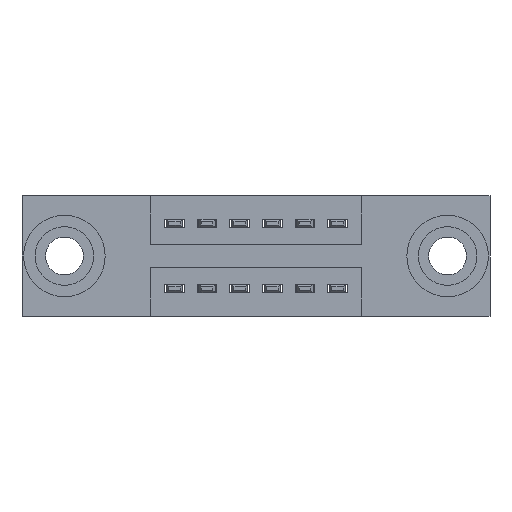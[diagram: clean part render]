
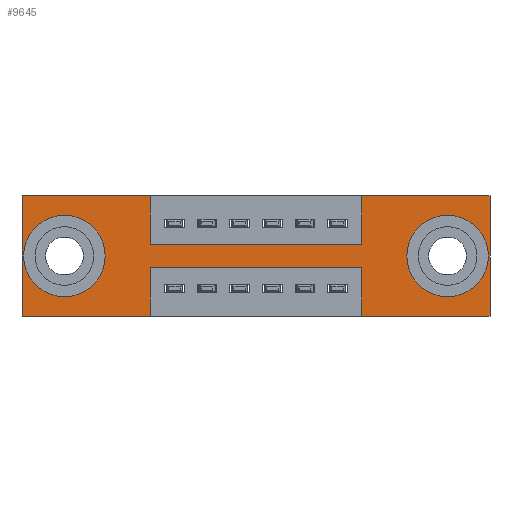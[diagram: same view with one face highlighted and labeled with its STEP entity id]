
A CAD part, front view. The second image highlights one B-rep face of the part: STEP entity #9645.
In plain terms, the highlighted planar face has unit normal (0, -1, 0).
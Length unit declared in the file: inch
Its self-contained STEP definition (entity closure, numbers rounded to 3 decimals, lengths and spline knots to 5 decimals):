
#14 = VERTEX_POINT ( 'NONE', #7489 ) ;
#21 = VECTOR ( 'NONE', #7703, 39.37008 ) ;
#127 = VERTEX_POINT ( 'NONE', #4537 ) ;
#397 = LINE ( 'NONE', #4495, #6055 ) ;
#702 = CARTESIAN_POINT ( 'NONE',  ( 0., 0., -0.37 ) ) ;
#749 = VECTOR ( 'NONE', #4626, 39.37008 ) ;
#845 = DIRECTION ( 'NONE',  ( 0., 0., 1. ) ) ;
#919 = DIRECTION ( 'NONE',  ( 0., 1., 0. ) ) ;
#989 = VERTEX_POINT ( 'NONE', #2778 ) ;
#1026 = LINE ( 'NONE', #3140, #4791 ) ;
#1046 = DIRECTION ( 'NONE',  ( 0., 0., -1. ) ) ;
#1113 = LINE ( 'NONE', #6927, #8847 ) ;
#1201 = DIRECTION ( 'NONE',  ( 0., 0., -1. ) ) ;
#1492 = ORIENTED_EDGE ( 'NONE', *, *, #8970, .F. ) ;
#1616 = VECTOR ( 'NONE', #5543, 39.37008 ) ;
#1700 = FACE_BOUND ( 'NONE', #3421, .T. ) ;
#1702 = ORIENTED_EDGE ( 'NONE', *, *, #8540, .T. ) ;
#1722 = CIRCLE ( 'NONE', #2268, 0.078 ) ;
#1865 = AXIS2_PLACEMENT_3D ( 'NONE', #5554, #919, #6311 ) ;
#1942 = PLANE ( 'NONE',  #3237 ) ;
#2005 = VERTEX_POINT ( 'NONE', #9450 ) ;
#2013 = AXIS2_PLACEMENT_3D ( 'NONE', #4120, #4902, #1046 ) ;
#2085 = CARTESIAN_POINT ( 'NONE',  ( 0., 0., 0. ) ) ;
#2108 = LINE ( 'NONE', #3737, #1616 ) ;
#2268 = AXIS2_PLACEMENT_3D ( 'NONE', #8088, #8887, #4190 ) ;
#2319 = DIRECTION ( 'NONE',  ( 0., 0., -1. ) ) ;
#2701 = VECTOR ( 'NONE', #6085, 39.37008 ) ;
#2749 = DIRECTION ( 'NONE',  ( 0., -1., 0. ) ) ;
#2778 = CARTESIAN_POINT ( 'NONE',  ( 1.435, 0., -0.37 ) ) ;
#2894 = ORIENTED_EDGE ( 'NONE', *, *, #7302, .F. ) ;
#3048 = EDGE_CURVE ( 'NONE', #7345, #127, #9031, .T. ) ;
#3110 = CARTESIAN_POINT ( 'NONE',  ( 0.13, 0., -0.263 ) ) ;
#3140 = CARTESIAN_POINT ( 'NONE',  ( 1.0425, 0., 0. ) ) ;
#3148 = FACE_BOUND ( 'NONE', #8759, .T. ) ;
#3237 = AXIS2_PLACEMENT_3D ( 'NONE', #5823, #2749, #1201 ) ;
#3384 = LINE ( 'NONE', #7835, #21 ) ;
#3421 = EDGE_LOOP ( 'NONE', ( #7200, #1702 ) ) ;
#3453 = CARTESIAN_POINT ( 'NONE',  ( 1.0425, 0., -0.22 ) ) ;
#3467 = CARTESIAN_POINT ( 'NONE',  ( 0., 0., 0. ) ) ;
#3473 = EDGE_CURVE ( 'NONE', #2005, #4674, #1026, .T. ) ;
#3604 = EDGE_CURVE ( 'NONE', #127, #7345, #7560, .T. ) ;
#3635 = CARTESIAN_POINT ( 'NONE',  ( 1.0425, 0., 0. ) ) ;
#3707 = CARTESIAN_POINT ( 'NONE',  ( 1.305, 0., -0.185 ) ) ;
#3736 = CARTESIAN_POINT ( 'NONE',  ( 0.3925, 0., -0.15 ) ) ;
#3737 = CARTESIAN_POINT ( 'NONE',  ( 0., 0., 0. ) ) ;
#3738 = DIRECTION ( 'NONE',  ( 0., 0., -1. ) ) ;
#3801 = VERTEX_POINT ( 'NONE', #10041 ) ;
#3845 = CARTESIAN_POINT ( 'NONE',  ( 0.3925, 0., 0. ) ) ;
#3860 = VERTEX_POINT ( 'NONE', #5006 ) ;
#3964 = ORIENTED_EDGE ( 'NONE', *, *, #8935, .F. ) ;
#4093 = ORIENTED_EDGE ( 'NONE', *, *, #7135, .F. ) ;
#4120 = CARTESIAN_POINT ( 'NONE',  ( 1.305, 0., -0.185 ) ) ;
#4127 = CARTESIAN_POINT ( 'NONE',  ( 1.435, 0., 0. ) ) ;
#4190 = DIRECTION ( 'NONE',  ( 0., 0., 1. ) ) ;
#4197 = CARTESIAN_POINT ( 'NONE',  ( 0.3925, 0., 0. ) ) ;
#4222 = ORIENTED_EDGE ( 'NONE', *, *, #7178, .F. ) ;
#4417 = VECTOR ( 'NONE', #6828, 39.37008 ) ;
#4495 = CARTESIAN_POINT ( 'NONE',  ( 1.435, 0., 0. ) ) ;
#4537 = CARTESIAN_POINT ( 'NONE',  ( 1.305, 0., -0.263 ) ) ;
#4626 = DIRECTION ( 'NONE',  ( 0., 0., -1. ) ) ;
#4647 = EDGE_CURVE ( 'NONE', #3801, #2005, #6429, .T. ) ;
#4674 = VERTEX_POINT ( 'NONE', #3635 ) ;
#4726 = ORIENTED_EDGE ( 'NONE', *, *, #3048, .T. ) ;
#4761 = LINE ( 'NONE', #10022, #2701 ) ;
#4791 = VECTOR ( 'NONE', #845, 39.37008 ) ;
#4902 = DIRECTION ( 'NONE',  ( 0., 1., 0. ) ) ;
#5006 = CARTESIAN_POINT ( 'NONE',  ( 0.3925, 0., -0.22 ) ) ;
#5101 = EDGE_CURVE ( 'NONE', #6743, #7125, #5962, .T. ) ;
#5230 = VERTEX_POINT ( 'NONE', #3110 ) ;
#5314 = EDGE_CURVE ( 'NONE', #989, #9769, #9468, .T. ) ;
#5410 = ORIENTED_EDGE ( 'NONE', *, *, #9427, .F. ) ;
#5413 = EDGE_CURVE ( 'NONE', #3860, #6776, #1113, .T. ) ;
#5426 = ORIENTED_EDGE ( 'NONE', *, *, #5413, .F. ) ;
#5447 = FACE_OUTER_BOUND ( 'NONE', #8054, .T. ) ;
#5543 = DIRECTION ( 'NONE',  ( 0., 0., 1. ) ) ;
#5551 = ORIENTED_EDGE ( 'NONE', *, *, #3604, .T. ) ;
#5554 = CARTESIAN_POINT ( 'NONE',  ( 0.13, 0., -0.185 ) ) ;
#5560 = CARTESIAN_POINT ( 'NONE',  ( 1.305, 0., -0.107 ) ) ;
#5597 = VECTOR ( 'NONE', #7647, 39.37008 ) ;
#5735 = CIRCLE ( 'NONE', #1865, 0.078 ) ;
#5823 = CARTESIAN_POINT ( 'NONE',  ( 0., 0., -0.37 ) ) ;
#5962 = LINE ( 'NONE', #3467, #9977 ) ;
#6055 = VECTOR ( 'NONE', #9184, 39.37008 ) ;
#6085 = DIRECTION ( 'NONE',  ( 0., 0., 1. ) ) ;
#6293 = VECTOR ( 'NONE', #7999, 39.37008 ) ;
#6311 = DIRECTION ( 'NONE',  ( 0., 0., 1. ) ) ;
#6429 = LINE ( 'NONE', #3736, #4417 ) ;
#6546 = CARTESIAN_POINT ( 'NONE',  ( 0.13, 0., -0.107 ) ) ;
#6661 = LINE ( 'NONE', #3845, #749 ) ;
#6692 = LINE ( 'NONE', #9579, #7045 ) ;
#6732 = CARTESIAN_POINT ( 'NONE',  ( 0., 0., 0. ) ) ;
#6743 = VERTEX_POINT ( 'NONE', #2085 ) ;
#6776 = VERTEX_POINT ( 'NONE', #9772 ) ;
#6828 = DIRECTION ( 'NONE',  ( 1., 0., 0. ) ) ;
#6927 = CARTESIAN_POINT ( 'NONE',  ( 0.3925, 0., -0.37 ) ) ;
#6940 = ORIENTED_EDGE ( 'NONE', *, *, #3473, .F. ) ;
#7045 = VECTOR ( 'NONE', #7358, 39.37008 ) ;
#7106 = EDGE_CURVE ( 'NONE', #9655, #5230, #5735, .T. ) ;
#7125 = VERTEX_POINT ( 'NONE', #4197 ) ;
#7135 = EDGE_CURVE ( 'NONE', #6776, #14, #6692, .T. ) ;
#7178 = EDGE_CURVE ( 'NONE', #14, #6743, #2108, .T. ) ;
#7200 = ORIENTED_EDGE ( 'NONE', *, *, #7106, .T. ) ;
#7265 = DIRECTION ( 'NONE',  ( 1., 0., 0. ) ) ;
#7302 = EDGE_CURVE ( 'NONE', #9769, #9454, #4761, .T. ) ;
#7345 = VERTEX_POINT ( 'NONE', #5560 ) ;
#7358 = DIRECTION ( 'NONE',  ( -1., 0., 0. ) ) ;
#7489 = CARTESIAN_POINT ( 'NONE',  ( 0., 0., -0.37 ) ) ;
#7536 = AXIS2_PLACEMENT_3D ( 'NONE', #3707, #7580, #3738 ) ;
#7560 = CIRCLE ( 'NONE', #7536, 0.078 ) ;
#7580 = DIRECTION ( 'NONE',  ( 0., 1., 0. ) ) ;
#7592 = ORIENTED_EDGE ( 'NONE', *, *, #9821, .F. ) ;
#7647 = DIRECTION ( 'NONE',  ( -1., 0., 0. ) ) ;
#7703 = DIRECTION ( 'NONE',  ( -1., 0., 0. ) ) ;
#7835 = CARTESIAN_POINT ( 'NONE',  ( 0.3925, 0., -0.22 ) ) ;
#7999 = DIRECTION ( 'NONE',  ( 1., 0., 0. ) ) ;
#8054 = EDGE_LOOP ( 'NONE', ( #5426, #7592, #2894, #8964, #3964, #1492, #6940, #9923, #5410, #8285, #4222, #4093 ) ) ;
#8088 = CARTESIAN_POINT ( 'NONE',  ( 0.13, 0., -0.185 ) ) ;
#8103 = LINE ( 'NONE', #6732, #6293 ) ;
#8285 = ORIENTED_EDGE ( 'NONE', *, *, #5101, .F. ) ;
#8540 = EDGE_CURVE ( 'NONE', #5230, #9655, #1722, .T. ) ;
#8759 = EDGE_LOOP ( 'NONE', ( #4726, #5551 ) ) ;
#8847 = VECTOR ( 'NONE', #2319, 39.37008 ) ;
#8887 = DIRECTION ( 'NONE',  ( 0., 1., 0. ) ) ;
#8935 = EDGE_CURVE ( 'NONE', #9512, #989, #397, .T. ) ;
#8964 = ORIENTED_EDGE ( 'NONE', *, *, #5314, .F. ) ;
#8970 = EDGE_CURVE ( 'NONE', #4674, #9512, #8103, .T. ) ;
#9031 = CIRCLE ( 'NONE', #2013, 0.078 ) ;
#9184 = DIRECTION ( 'NONE',  ( 0., 0., -1. ) ) ;
#9307 = CARTESIAN_POINT ( 'NONE',  ( 1.0425, 0., -0.37 ) ) ;
#9427 = EDGE_CURVE ( 'NONE', #7125, #3801, #6661, .T. ) ;
#9450 = CARTESIAN_POINT ( 'NONE',  ( 1.0425, 0., -0.15 ) ) ;
#9454 = VERTEX_POINT ( 'NONE', #3453 ) ;
#9468 = LINE ( 'NONE', #702, #5597 ) ;
#9512 = VERTEX_POINT ( 'NONE', #4127 ) ;
#9579 = CARTESIAN_POINT ( 'NONE',  ( 0., 0., -0.37 ) ) ;
#9645 = ADVANCED_FACE ( 'NONE', ( #3148, #1700, #5447 ), #1942, .T. ) ;
#9655 = VERTEX_POINT ( 'NONE', #6546 ) ;
#9769 = VERTEX_POINT ( 'NONE', #9307 ) ;
#9772 = CARTESIAN_POINT ( 'NONE',  ( 0.3925, 0., -0.37 ) ) ;
#9821 = EDGE_CURVE ( 'NONE', #9454, #3860, #3384, .T. ) ;
#9923 = ORIENTED_EDGE ( 'NONE', *, *, #4647, .F. ) ;
#9977 = VECTOR ( 'NONE', #7265, 39.37008 ) ;
#10022 = CARTESIAN_POINT ( 'NONE',  ( 1.0425, 0., -0.37 ) ) ;
#10041 = CARTESIAN_POINT ( 'NONE',  ( 0.3925, 0., -0.15 ) ) ;
